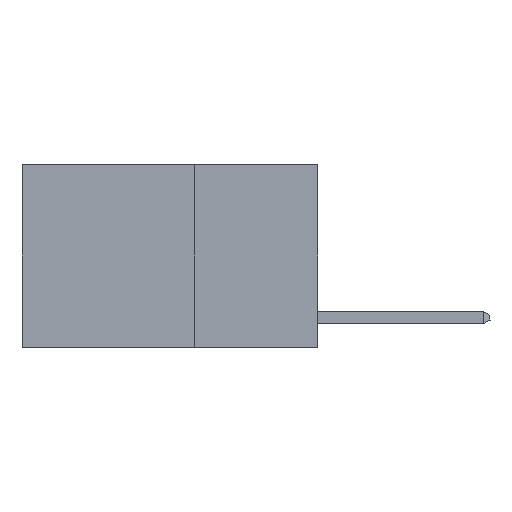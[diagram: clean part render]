
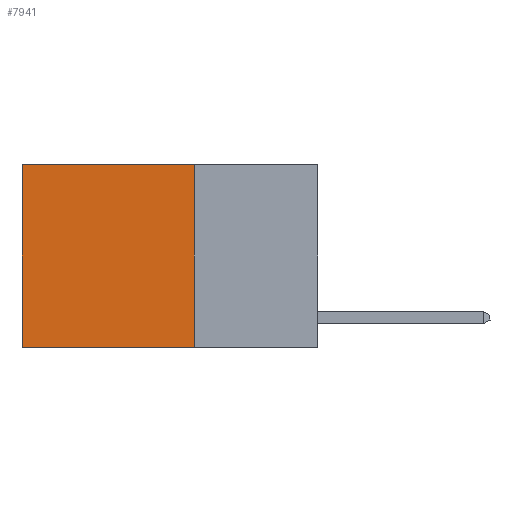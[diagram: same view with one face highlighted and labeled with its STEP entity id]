
A CAD part, left-side view. The second image highlights one B-rep face of the part: STEP entity #7941.
In plain terms, the highlighted planar face has unit normal (-1, 0, 0).
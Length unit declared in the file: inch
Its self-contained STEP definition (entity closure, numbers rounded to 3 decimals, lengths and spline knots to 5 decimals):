
#918 = ORIENTED_EDGE ( 'NONE', *, *, #9177, .T. ) ;
#977 = EDGE_CURVE ( 'NONE', #4578, #4701, #6669, .T. ) ;
#1259 = CARTESIAN_POINT ( 'NONE',  ( 0.2625, 0.25, -0.37 ) ) ;
#1487 = CARTESIAN_POINT ( 'NONE',  ( 0.2625, 0.25, 0. ) ) ;
#1675 = VECTOR ( 'NONE', #3354, 39.37008 ) ;
#1872 = CARTESIAN_POINT ( 'NONE',  ( 0.2625, 0.6, -0.37 ) ) ;
#2431 = PLANE ( 'NONE',  #6583 ) ;
#3175 = EDGE_LOOP ( 'NONE', ( #4869, #6914, #8873, #918 ) ) ;
#3239 = VECTOR ( 'NONE', #4895, 39.37008 ) ;
#3354 = DIRECTION ( 'NONE',  ( 0., 1., 0. ) ) ;
#3773 = LINE ( 'NONE', #4889, #1675 ) ;
#4078 = CARTESIAN_POINT ( 'NONE',  ( 0.2625, 0.6, 0. ) ) ;
#4381 = VECTOR ( 'NONE', #5825, 39.37008 ) ;
#4578 = VERTEX_POINT ( 'NONE', #4078 ) ;
#4701 = VERTEX_POINT ( 'NONE', #1872 ) ;
#4765 = CARTESIAN_POINT ( 'NONE',  ( 0.2625, 0.25, 0. ) ) ;
#4800 = DIRECTION ( 'NONE',  ( 1., 0., 0. ) ) ;
#4869 = ORIENTED_EDGE ( 'NONE', *, *, #977, .T. ) ;
#4889 = CARTESIAN_POINT ( 'NONE',  ( 0.2625, 0.25, 0. ) ) ;
#4895 = DIRECTION ( 'NONE',  ( 0., 1., 0. ) ) ;
#4931 = CARTESIAN_POINT ( 'NONE',  ( 0.2625, 0.25, -0.37 ) ) ;
#5537 = LINE ( 'NONE', #4931, #3239 ) ;
#5621 = VERTEX_POINT ( 'NONE', #1259 ) ;
#5808 = LINE ( 'NONE', #1487, #7376 ) ;
#5825 = DIRECTION ( 'NONE',  ( 0., 0., -1. ) ) ;
#5925 = CARTESIAN_POINT ( 'NONE',  ( 0.2625, 0.6, 0. ) ) ;
#6495 = FACE_OUTER_BOUND ( 'NONE', #3175, .T. ) ;
#6583 = AXIS2_PLACEMENT_3D ( 'NONE', #4765, #4800, #10029 ) ;
#6669 = LINE ( 'NONE', #5925, #4381 ) ;
#6914 = ORIENTED_EDGE ( 'NONE', *, *, #8079, .F. ) ;
#7376 = VECTOR ( 'NONE', #9866, 39.37008 ) ;
#7941 = ADVANCED_FACE ( 'NONE', ( #6495 ), #2431, .F. ) ;
#8079 = EDGE_CURVE ( 'NONE', #5621, #4701, #5537, .T. ) ;
#8343 = CARTESIAN_POINT ( 'NONE',  ( 0.2625, 0.25, 0. ) ) ;
#8413 = VERTEX_POINT ( 'NONE', #8343 ) ;
#8873 = ORIENTED_EDGE ( 'NONE', *, *, #9654, .F. ) ;
#9177 = EDGE_CURVE ( 'NONE', #8413, #4578, #3773, .T. ) ;
#9654 = EDGE_CURVE ( 'NONE', #8413, #5621, #5808, .T. ) ;
#9866 = DIRECTION ( 'NONE',  ( 0., 0., -1. ) ) ;
#10029 = DIRECTION ( 'NONE',  ( 0., 0., -1. ) ) ;
